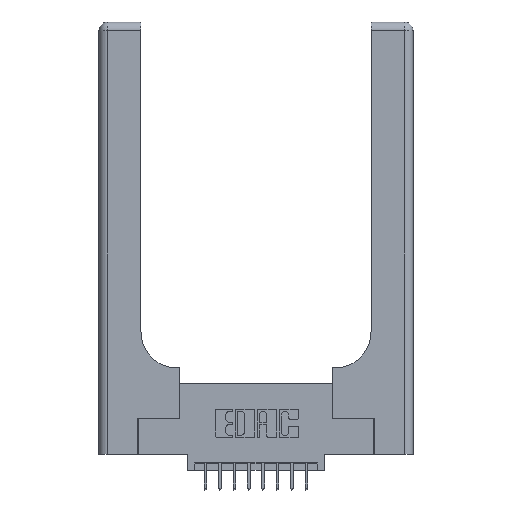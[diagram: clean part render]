
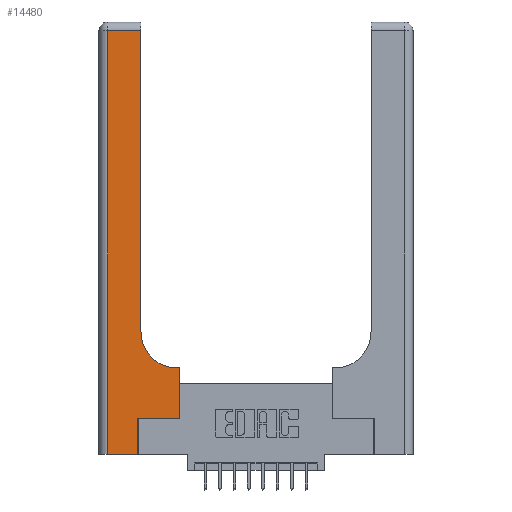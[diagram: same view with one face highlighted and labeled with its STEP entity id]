
A CAD part, top view. The second image highlights one B-rep face of the part: STEP entity #14480.
In plain terms, the highlighted planar face has unit normal (0, 0, 1).
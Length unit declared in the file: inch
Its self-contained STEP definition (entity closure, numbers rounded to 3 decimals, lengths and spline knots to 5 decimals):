
#23 = VERTEX_POINT ( 'NONE', #2012 ) ;
#373 = CARTESIAN_POINT ( 'NONE',  ( 0.06, 3., 0.37 ) ) ;
#378 = VERTEX_POINT ( 'NONE', #1370 ) ;
#688 = CARTESIAN_POINT ( 'NONE',  ( 0.5415, 0.6, 0.37 ) ) ;
#1049 = VECTOR ( 'NONE', #14547, 39.37008 ) ;
#1369 = LINE ( 'NONE', #11418, #7812 ) ;
#1370 = CARTESIAN_POINT ( 'NONE',  ( 0.269, 0.25, 0.37 ) ) ;
#1415 = ORIENTED_EDGE ( 'NONE', *, *, #9694, .T. ) ;
#1549 = DIRECTION ( 'NONE',  ( 1., 0., 0. ) ) ;
#1680 = CARTESIAN_POINT ( 'NONE',  ( 0., 2.94, 0.37 ) ) ;
#1717 = LINE ( 'NONE', #9481, #1049 ) ;
#1899 = DIRECTION ( 'NONE',  ( 0., 1., 0. ) ) ;
#1926 = CARTESIAN_POINT ( 'NONE',  ( 0.5585, 0.6, 0.37 ) ) ;
#2012 = CARTESIAN_POINT ( 'NONE',  ( 0.269, 0., 0.37 ) ) ;
#2087 = VERTEX_POINT ( 'NONE', #688 ) ;
#2373 = AXIS2_PLACEMENT_3D ( 'NONE', #13700, #13540, #8475 ) ;
#2387 = CIRCLE ( 'NONE', #2373, 0.25 ) ;
#2434 = VECTOR ( 'NONE', #1899, 39.37008 ) ;
#2441 = LINE ( 'NONE', #7495, #7521 ) ;
#2488 = EDGE_LOOP ( 'NONE', ( #5087, #7997, #7226, #5787, #3984, #13730, #1415, #13993, #12588 ) ) ;
#2884 = LINE ( 'NONE', #1680, #7284 ) ;
#3516 = CARTESIAN_POINT ( 'NONE',  ( 0.5585, 0.25, 0.37 ) ) ;
#3653 = PLANE ( 'NONE',  #9947 ) ;
#3730 = DIRECTION ( 'NONE',  ( 1., 0., 0. ) ) ;
#3828 = DIRECTION ( 'NONE',  ( -1., 0., 0. ) ) ;
#3984 = ORIENTED_EDGE ( 'NONE', *, *, #7106, .T. ) ;
#4309 = LINE ( 'NONE', #7822, #15222 ) ;
#4538 = EDGE_CURVE ( 'NONE', #2087, #9657, #2387, .T. ) ;
#4760 = VERTEX_POINT ( 'NONE', #1926 ) ;
#5020 = CARTESIAN_POINT ( 'NONE',  ( 0.2915, 2.94, 0.37 ) ) ;
#5087 = ORIENTED_EDGE ( 'NONE', *, *, #15890, .T. ) ;
#5787 = ORIENTED_EDGE ( 'NONE', *, *, #15117, .T. ) ;
#6616 = LINE ( 'NONE', #373, #7826 ) ;
#6688 = DIRECTION ( 'NONE',  ( -1., 0., 0. ) ) ;
#7106 = EDGE_CURVE ( 'NONE', #23, #378, #9126, .T. ) ;
#7226 = ORIENTED_EDGE ( 'NONE', *, *, #10385, .T. ) ;
#7284 = VECTOR ( 'NONE', #6688, 39.37008 ) ;
#7495 = CARTESIAN_POINT ( 'NONE',  ( 0.5585, 0.25, 0.37 ) ) ;
#7521 = VECTOR ( 'NONE', #15057, 39.37008 ) ;
#7768 = VERTEX_POINT ( 'NONE', #14349 ) ;
#7812 = VECTOR ( 'NONE', #3730, 39.37008 ) ;
#7822 = CARTESIAN_POINT ( 'NONE',  ( 0., 0., 0.37 ) ) ;
#7826 = VECTOR ( 'NONE', #10427, 39.37008 ) ;
#7997 = ORIENTED_EDGE ( 'NONE', *, *, #10662, .T. ) ;
#8475 = DIRECTION ( 'NONE',  ( 1., 0., 0. ) ) ;
#8568 = VERTEX_POINT ( 'NONE', #5020 ) ;
#9126 = LINE ( 'NONE', #13177, #2434 ) ;
#9481 = CARTESIAN_POINT ( 'NONE',  ( 0.2915, 0.6, 0.37 ) ) ;
#9657 = VERTEX_POINT ( 'NONE', #12263 ) ;
#9694 = EDGE_CURVE ( 'NONE', #9957, #4760, #2441, .T. ) ;
#9947 = AXIS2_PLACEMENT_3D ( 'NONE', #15110, #11006, #3828 ) ;
#9957 = VERTEX_POINT ( 'NONE', #3516 ) ;
#10282 = EDGE_CURVE ( 'NONE', #378, #9957, #1369, .T. ) ;
#10385 = EDGE_CURVE ( 'NONE', #7768, #13620, #6616, .T. ) ;
#10427 = DIRECTION ( 'NONE',  ( 0., -1., 0. ) ) ;
#10493 = CARTESIAN_POINT ( 'NONE',  ( 0.2915, 3., 0.37 ) ) ;
#10566 = DIRECTION ( 'NONE',  ( 0., 1., 0. ) ) ;
#10662 = EDGE_CURVE ( 'NONE', #8568, #7768, #2884, .T. ) ;
#11006 = DIRECTION ( 'NONE',  ( 0., 0., -1. ) ) ;
#11418 = CARTESIAN_POINT ( 'NONE',  ( 0.269, 0.25, 0.37 ) ) ;
#11814 = VECTOR ( 'NONE', #10566, 39.37008 ) ;
#12263 = CARTESIAN_POINT ( 'NONE',  ( 0.2915, 0.85, 0.37 ) ) ;
#12588 = ORIENTED_EDGE ( 'NONE', *, *, #4538, .T. ) ;
#13121 = LINE ( 'NONE', #10493, #11814 ) ;
#13177 = CARTESIAN_POINT ( 'NONE',  ( 0.269, 0., 0.37 ) ) ;
#13540 = DIRECTION ( 'NONE',  ( 0., 0., -1. ) ) ;
#13620 = VERTEX_POINT ( 'NONE', #14287 ) ;
#13700 = CARTESIAN_POINT ( 'NONE',  ( 0.5415, 0.85, 0.37 ) ) ;
#13730 = ORIENTED_EDGE ( 'NONE', *, *, #10282, .T. ) ;
#13798 = FACE_OUTER_BOUND ( 'NONE', #2488, .T. ) ;
#13993 = ORIENTED_EDGE ( 'NONE', *, *, #16190, .T. ) ;
#14287 = CARTESIAN_POINT ( 'NONE',  ( 0.06, 0., 0.37 ) ) ;
#14349 = CARTESIAN_POINT ( 'NONE',  ( 0.06, 2.94, 0.37 ) ) ;
#14480 = ADVANCED_FACE ( 'NONE', ( #13798 ), #3653, .F. ) ;
#14547 = DIRECTION ( 'NONE',  ( -1., 0., 0. ) ) ;
#15057 = DIRECTION ( 'NONE',  ( 0., 1., 0. ) ) ;
#15110 = CARTESIAN_POINT ( 'NONE',  ( 0., 3., 0.37 ) ) ;
#15117 = EDGE_CURVE ( 'NONE', #13620, #23, #4309, .T. ) ;
#15222 = VECTOR ( 'NONE', #1549, 39.37008 ) ;
#15890 = EDGE_CURVE ( 'NONE', #9657, #8568, #13121, .T. ) ;
#16190 = EDGE_CURVE ( 'NONE', #4760, #2087, #1717, .T. ) ;
